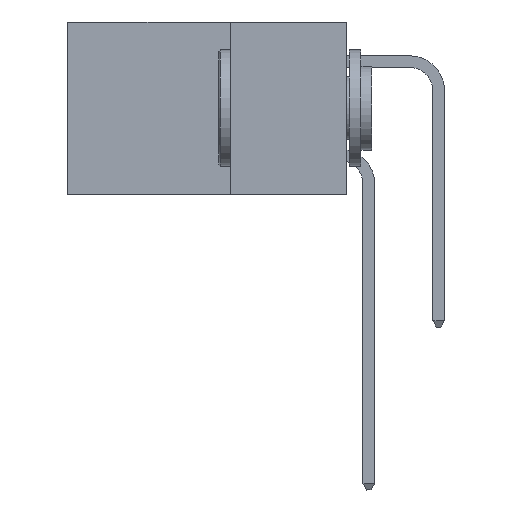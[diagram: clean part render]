
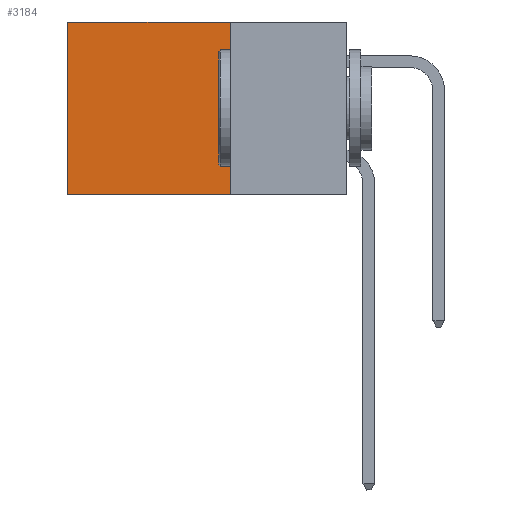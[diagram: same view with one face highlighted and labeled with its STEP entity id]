
A CAD part, left-side view. The second image highlights one B-rep face of the part: STEP entity #3184.
In plain terms, the highlighted planar face has unit normal (-1, 0, 0).
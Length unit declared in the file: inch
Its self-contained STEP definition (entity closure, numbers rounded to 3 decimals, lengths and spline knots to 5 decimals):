
#451 = EDGE_CURVE ( 'NONE', #28634, #16036, #32644, .T. ) ;
#1995 = LINE ( 'NONE', #15248, #23691 ) ;
#3184 = ADVANCED_FACE ( 'NONE', ( #8320 ), #24926, .F. ) ;
#3444 = EDGE_CURVE ( 'NONE', #34158, #15620, #1995, .T. ) ;
#6056 = DIRECTION ( 'NONE',  ( 1., 0., 0. ) ) ;
#7820 = CARTESIAN_POINT ( 'NONE',  ( 0.2875, 0.25, 0. ) ) ;
#8320 = FACE_OUTER_BOUND ( 'NONE', #33038, .T. ) ;
#8451 = ORIENTED_EDGE ( 'NONE', *, *, #451, .F. ) ;
#10568 = CARTESIAN_POINT ( 'NONE',  ( 0.2875, 0.25, 0. ) ) ;
#10852 = LINE ( 'NONE', #33315, #18996 ) ;
#12129 = CARTESIAN_POINT ( 'NONE',  ( 0.2875, 0.25, -0.37 ) ) ;
#13079 = DIRECTION ( 'NONE',  ( 0., 1., 0. ) ) ;
#15248 = CARTESIAN_POINT ( 'NONE',  ( 0.2875, 0.6, 0. ) ) ;
#15620 = VERTEX_POINT ( 'NONE', #20959 ) ;
#16036 = VERTEX_POINT ( 'NONE', #12129 ) ;
#16087 = AXIS2_PLACEMENT_3D ( 'NONE', #27779, #6056, #27899 ) ;
#16273 = EDGE_CURVE ( 'NONE', #28634, #34158, #18824, .T. ) ;
#18824 = LINE ( 'NONE', #10568, #27342 ) ;
#18996 = VECTOR ( 'NONE', #30699, 39.37008 ) ;
#20959 = CARTESIAN_POINT ( 'NONE',  ( 0.2875, 0.6, -0.37 ) ) ;
#21311 = ORIENTED_EDGE ( 'NONE', *, *, #3444, .T. ) ;
#22314 = CARTESIAN_POINT ( 'NONE',  ( 0.2875, 0.25, 0. ) ) ;
#22946 = ORIENTED_EDGE ( 'NONE', *, *, #16273, .T. ) ;
#23691 = VECTOR ( 'NONE', #34343, 39.37008 ) ;
#24926 = PLANE ( 'NONE',  #16087 ) ;
#26684 = DIRECTION ( 'NONE',  ( 0., 0., -1. ) ) ;
#27084 = VECTOR ( 'NONE', #26684, 39.37008 ) ;
#27342 = VECTOR ( 'NONE', #13079, 39.37008 ) ;
#27779 = CARTESIAN_POINT ( 'NONE',  ( 0.2875, 0.25, 0. ) ) ;
#27899 = DIRECTION ( 'NONE',  ( 0., 0., -1. ) ) ;
#28072 = CARTESIAN_POINT ( 'NONE',  ( 0.2875, 0.6, 0. ) ) ;
#28634 = VERTEX_POINT ( 'NONE', #22314 ) ;
#30699 = DIRECTION ( 'NONE',  ( 0., 1., 0. ) ) ;
#31268 = EDGE_CURVE ( 'NONE', #16036, #15620, #10852, .T. ) ;
#32644 = LINE ( 'NONE', #7820, #27084 ) ;
#33038 = EDGE_LOOP ( 'NONE', ( #21311, #33599, #8451, #22946 ) ) ;
#33315 = CARTESIAN_POINT ( 'NONE',  ( 0.2875, 0.25, -0.37 ) ) ;
#33599 = ORIENTED_EDGE ( 'NONE', *, *, #31268, .F. ) ;
#34158 = VERTEX_POINT ( 'NONE', #28072 ) ;
#34343 = DIRECTION ( 'NONE',  ( 0., 0., -1. ) ) ;
